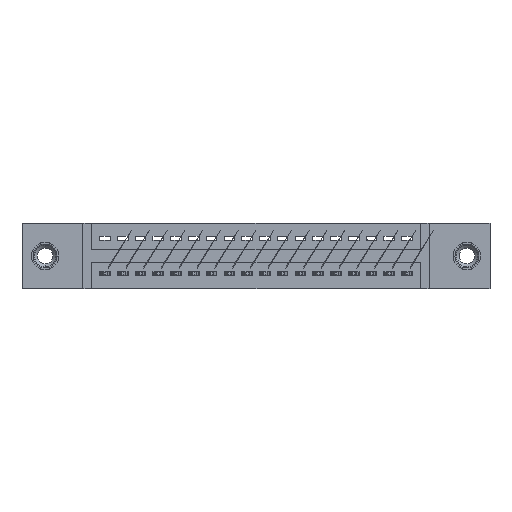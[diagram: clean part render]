
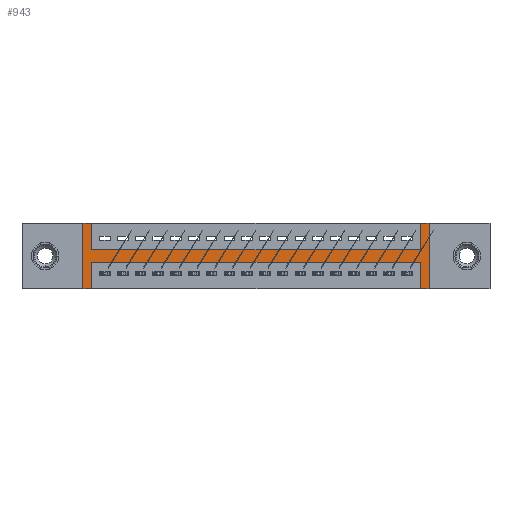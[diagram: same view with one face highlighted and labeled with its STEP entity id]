
A CAD part, front view. The second image highlights one B-rep face of the part: STEP entity #943.
In plain terms, the highlighted planar face has unit normal (0, -1, 0).
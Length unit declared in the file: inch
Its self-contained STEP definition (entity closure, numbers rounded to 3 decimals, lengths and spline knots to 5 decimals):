
#245 = VERTEX_POINT ( 'NONE', #18087 ) ;
#375 = DIRECTION ( 'NONE',  ( -1., 0., 0. ) ) ;
#568 = LINE ( 'NONE', #2801, #7220 ) ;
#727 = CARTESIAN_POINT ( 'NONE',  ( 0., 0., -0.37 ) ) ;
#750 = CARTESIAN_POINT ( 'NONE',  ( 2.2925, 0., 0. ) ) ;
#943 = ADVANCED_FACE ( 'NONE', ( #13295 ), #9138, .T. ) ;
#1331 = LINE ( 'NONE', #16854, #7946 ) ;
#1636 = VECTOR ( 'NONE', #5822, 39.37008 ) ;
#1843 = AXIS2_PLACEMENT_3D ( 'NONE', #6319, #3170, #18089 ) ;
#2068 = VECTOR ( 'NONE', #2426, 39.37008 ) ;
#2177 = CARTESIAN_POINT ( 'NONE',  ( 0., 0., 0. ) ) ;
#2426 = DIRECTION ( 'NONE',  ( 0., 0., 1. ) ) ;
#2526 = LINE ( 'NONE', #750, #16905 ) ;
#2661 = ORIENTED_EDGE ( 'NONE', *, *, #6929, .F. ) ;
#2801 = CARTESIAN_POINT ( 'NONE',  ( 0., 0., 0. ) ) ;
#2917 = EDGE_CURVE ( 'NONE', #245, #2955, #6183, .T. ) ;
#2955 = VERTEX_POINT ( 'NONE', #5316 ) ;
#2976 = CARTESIAN_POINT ( 'NONE',  ( 0.3925, 0., -0.22 ) ) ;
#3170 = DIRECTION ( 'NONE',  ( 0., -1., 0. ) ) ;
#3214 = CARTESIAN_POINT ( 'NONE',  ( 2.2925, 0., -0.37 ) ) ;
#3260 = CARTESIAN_POINT ( 'NONE',  ( 0.3425, 0., 0. ) ) ;
#3305 = VERTEX_POINT ( 'NONE', #6090 ) ;
#3932 = VERTEX_POINT ( 'NONE', #12929 ) ;
#4287 = VERTEX_POINT ( 'NONE', #15041 ) ;
#4395 = EDGE_CURVE ( 'NONE', #8723, #7971, #568, .T. ) ;
#4552 = VECTOR ( 'NONE', #14769, 39.37008 ) ;
#4994 = LINE ( 'NONE', #2177, #4552 ) ;
#5316 = CARTESIAN_POINT ( 'NONE',  ( 0.3925, 0., -0.37 ) ) ;
#5435 = LINE ( 'NONE', #2976, #1636 ) ;
#5450 = EDGE_CURVE ( 'NONE', #4287, #6327, #4994, .T. ) ;
#5507 = EDGE_CURVE ( 'NONE', #7971, #3305, #18012, .T. ) ;
#5822 = DIRECTION ( 'NONE',  ( -1., 0., 0. ) ) ;
#6037 = CARTESIAN_POINT ( 'NONE',  ( 2.2425, 0., 0. ) ) ;
#6090 = CARTESIAN_POINT ( 'NONE',  ( 0.3925, 0., -0.15 ) ) ;
#6151 = CARTESIAN_POINT ( 'NONE',  ( 0.3925, 0., 0. ) ) ;
#6183 = LINE ( 'NONE', #13514, #17248 ) ;
#6200 = EDGE_CURVE ( 'NONE', #6327, #7902, #2526, .T. ) ;
#6261 = VECTOR ( 'NONE', #17131, 39.37008 ) ;
#6319 = CARTESIAN_POINT ( 'NONE',  ( 0., 0., -0.37 ) ) ;
#6327 = VERTEX_POINT ( 'NONE', #10800 ) ;
#6464 = DIRECTION ( 'NONE',  ( 0., 0., -1. ) ) ;
#6554 = CARTESIAN_POINT ( 'NONE',  ( 2.2425, 0., -0.15 ) ) ;
#6824 = EDGE_CURVE ( 'NONE', #2955, #9119, #11439, .T. ) ;
#6929 = EDGE_CURVE ( 'NONE', #3932, #9951, #16908, .T. ) ;
#7220 = VECTOR ( 'NONE', #16722, 39.37008 ) ;
#7381 = EDGE_LOOP ( 'NONE', ( #12877, #12759, #12725, #12252, #12219, #12045, #11789, #12691, #11472, #9353, #2661, #11633 ) ) ;
#7717 = EDGE_CURVE ( 'NONE', #3305, #14225, #10046, .T. ) ;
#7902 = VERTEX_POINT ( 'NONE', #3214 ) ;
#7946 = VECTOR ( 'NONE', #9917, 39.37008 ) ;
#7971 = VERTEX_POINT ( 'NONE', #6151 ) ;
#7987 = DIRECTION ( 'NONE',  ( 0., 0., -1. ) ) ;
#8723 = VERTEX_POINT ( 'NONE', #3260 ) ;
#9119 = VERTEX_POINT ( 'NONE', #15357 ) ;
#9138 = PLANE ( 'NONE',  #1843 ) ;
#9353 = ORIENTED_EDGE ( 'NONE', *, *, #9814, .F. ) ;
#9376 = CARTESIAN_POINT ( 'NONE',  ( 2.2425, 0., -0.37 ) ) ;
#9814 = EDGE_CURVE ( 'NONE', #9951, #245, #5435, .T. ) ;
#9917 = DIRECTION ( 'NONE',  ( 0., 0., 1. ) ) ;
#9951 = VERTEX_POINT ( 'NONE', #13028 ) ;
#10046 = LINE ( 'NONE', #18046, #13335 ) ;
#10474 = EDGE_CURVE ( 'NONE', #7902, #3932, #11222, .T. ) ;
#10800 = CARTESIAN_POINT ( 'NONE',  ( 2.2925, 0., 0. ) ) ;
#11222 = LINE ( 'NONE', #14358, #14526 ) ;
#11439 = LINE ( 'NONE', #727, #15152 ) ;
#11472 = ORIENTED_EDGE ( 'NONE', *, *, #2917, .F. ) ;
#11633 = ORIENTED_EDGE ( 'NONE', *, *, #10474, .F. ) ;
#11789 = ORIENTED_EDGE ( 'NONE', *, *, #15732, .F. ) ;
#11933 = DIRECTION ( 'NONE',  ( -1., 0., 0. ) ) ;
#12045 = ORIENTED_EDGE ( 'NONE', *, *, #4395, .F. ) ;
#12219 = ORIENTED_EDGE ( 'NONE', *, *, #5507, .F. ) ;
#12252 = ORIENTED_EDGE ( 'NONE', *, *, #7717, .F. ) ;
#12691 = ORIENTED_EDGE ( 'NONE', *, *, #6824, .F. ) ;
#12725 = ORIENTED_EDGE ( 'NONE', *, *, #14577, .F. ) ;
#12759 = ORIENTED_EDGE ( 'NONE', *, *, #5450, .F. ) ;
#12877 = ORIENTED_EDGE ( 'NONE', *, *, #6200, .F. ) ;
#12929 = CARTESIAN_POINT ( 'NONE',  ( 2.2425, 0., -0.37 ) ) ;
#13028 = CARTESIAN_POINT ( 'NONE',  ( 2.2425, 0., -0.22 ) ) ;
#13295 = FACE_OUTER_BOUND ( 'NONE', #7381, .T. ) ;
#13335 = VECTOR ( 'NONE', #15266, 39.37008 ) ;
#13487 = CARTESIAN_POINT ( 'NONE',  ( 0.3925, 0., 0. ) ) ;
#13514 = CARTESIAN_POINT ( 'NONE',  ( 0.3925, 0., -0.37 ) ) ;
#14225 = VERTEX_POINT ( 'NONE', #6554 ) ;
#14358 = CARTESIAN_POINT ( 'NONE',  ( 0., 0., -0.37 ) ) ;
#14526 = VECTOR ( 'NONE', #375, 39.37008 ) ;
#14577 = EDGE_CURVE ( 'NONE', #14225, #4287, #17319, .T. ) ;
#14769 = DIRECTION ( 'NONE',  ( 1., 0., 0. ) ) ;
#14889 = DIRECTION ( 'NONE',  ( 0., 0., -1. ) ) ;
#15041 = CARTESIAN_POINT ( 'NONE',  ( 2.2425, 0., 0. ) ) ;
#15152 = VECTOR ( 'NONE', #11933, 39.37008 ) ;
#15266 = DIRECTION ( 'NONE',  ( 1., 0., 0. ) ) ;
#15357 = CARTESIAN_POINT ( 'NONE',  ( 0.3425, 0., -0.37 ) ) ;
#15732 = EDGE_CURVE ( 'NONE', #9119, #8723, #1331, .T. ) ;
#16722 = DIRECTION ( 'NONE',  ( 1., 0., 0. ) ) ;
#16854 = CARTESIAN_POINT ( 'NONE',  ( 0.3425, 0., 0. ) ) ;
#16905 = VECTOR ( 'NONE', #6464, 39.37008 ) ;
#16908 = LINE ( 'NONE', #9376, #2068 ) ;
#17131 = DIRECTION ( 'NONE',  ( 0., 0., 1. ) ) ;
#17248 = VECTOR ( 'NONE', #7987, 39.37008 ) ;
#17319 = LINE ( 'NONE', #6037, #6261 ) ;
#17569 = VECTOR ( 'NONE', #14889, 39.37008 ) ;
#18012 = LINE ( 'NONE', #13487, #17569 ) ;
#18046 = CARTESIAN_POINT ( 'NONE',  ( 0.3925, 0., -0.15 ) ) ;
#18087 = CARTESIAN_POINT ( 'NONE',  ( 0.3925, 0., -0.22 ) ) ;
#18089 = DIRECTION ( 'NONE',  ( 0., 0., -1. ) ) ;
